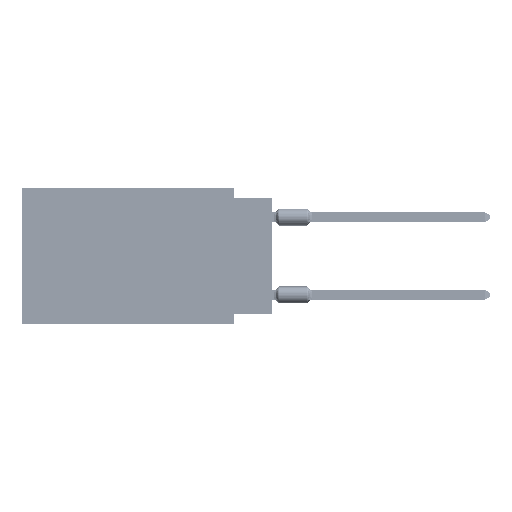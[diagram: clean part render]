
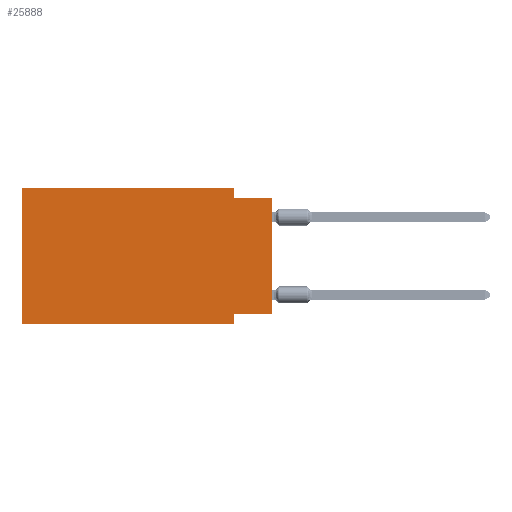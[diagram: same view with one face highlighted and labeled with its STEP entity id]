
A CAD part, left-side view. The second image highlights one B-rep face of the part: STEP entity #25888.
In plain terms, the highlighted planar face has unit normal (-1, 0, 0).
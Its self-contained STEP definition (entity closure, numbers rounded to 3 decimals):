
#6330 = VECTOR ( 'NONE', #55003, 1000. ) ;
#9241 = CARTESIAN_POINT ( 'NONE',  ( 0., 16.383, -8.89 ) ) ;
#10294 = EDGE_CURVE ( 'NONE', #30909, #75655, #40972, .T. ) ;
#11372 = ORIENTED_EDGE ( 'NONE', *, *, #43474, .F. ) ;
#11566 = LINE ( 'NONE', #36712, #68965 ) ;
#12037 = CARTESIAN_POINT ( 'NONE',  ( 0., 2.54, -8.89 ) ) ;
#12846 = LINE ( 'NONE', #12037, #32940 ) ;
#14534 = ORIENTED_EDGE ( 'NONE', *, *, #39581, .T. ) ;
#15841 = CARTESIAN_POINT ( 'NONE',  ( 0., 16.383, -8.89 ) ) ;
#17546 = VERTEX_POINT ( 'NONE', #73721 ) ;
#18106 = CARTESIAN_POINT ( 'NONE',  ( 0., 16.383, 0. ) ) ;
#19044 = VERTEX_POINT ( 'NONE', #76239 ) ;
#19432 = VERTEX_POINT ( 'NONE', #58290 ) ;
#19687 = LINE ( 'NONE', #53488, #44958 ) ;
#25888 = ADVANCED_FACE ( 'NONE', ( #49856 ), #80800, .F. ) ;
#26780 = VECTOR ( 'NONE', #71917, 1000. ) ;
#26903 = CARTESIAN_POINT ( 'NONE',  ( 0., 2.54, -8.89 ) ) ;
#28178 = CARTESIAN_POINT ( 'NONE',  ( 0., 16.383, 0. ) ) ;
#28678 = ORIENTED_EDGE ( 'NONE', *, *, #10294, .F. ) ;
#30092 = ORIENTED_EDGE ( 'NONE', *, *, #61820, .F. ) ;
#30909 = VERTEX_POINT ( 'NONE', #80794 ) ;
#31813 = DIRECTION ( 'NONE',  ( 0., 0., -1. ) ) ;
#32940 = VECTOR ( 'NONE', #31813, 1000. ) ;
#33059 = VECTOR ( 'NONE', #66560, 1000. ) ;
#33509 = CARTESIAN_POINT ( 'NONE',  ( 0., 16.383, 0. ) ) ;
#34720 = EDGE_CURVE ( 'NONE', #19432, #17546, #40091, .T. ) ;
#36712 = CARTESIAN_POINT ( 'NONE',  ( 0., 0., 0. ) ) ;
#38563 = DIRECTION ( 'NONE',  ( 0., -1., 0. ) ) ;
#38978 = VERTEX_POINT ( 'NONE', #26903 ) ;
#39581 = EDGE_CURVE ( 'NONE', #64849, #38978, #71942, .T. ) ;
#40091 = LINE ( 'NONE', #65261, #55985 ) ;
#40972 = LINE ( 'NONE', #66147, #33059 ) ;
#41267 = EDGE_LOOP ( 'NONE', ( #81431, #60183, #72199, #11372, #30092, #14534, #71300, #28678 ) ) ;
#43474 = EDGE_CURVE ( 'NONE', #45913, #19432, #19687, .T. ) ;
#43666 = DIRECTION ( 'NONE',  ( 0., 0., -1. ) ) ;
#44757 = CARTESIAN_POINT ( 'NONE',  ( 0., 0., -0.635 ) ) ;
#44958 = VECTOR ( 'NONE', #72061, 1000. ) ;
#45913 = VERTEX_POINT ( 'NONE', #33509 ) ;
#49856 = FACE_OUTER_BOUND ( 'NONE', #41267, .T. ) ;
#50536 = LINE ( 'NONE', #44757, #60083 ) ;
#53488 = CARTESIAN_POINT ( 'NONE',  ( 0., 16.383, 0. ) ) ;
#55003 = DIRECTION ( 'NONE',  ( 0., -1., 0. ) ) ;
#55685 = DIRECTION ( 'NONE',  ( 0., 0., 1. ) ) ;
#55985 = VECTOR ( 'NONE', #76825, 1000. ) ;
#58290 = CARTESIAN_POINT ( 'NONE',  ( 0., 2.54, 0. ) ) ;
#60073 = EDGE_CURVE ( 'NONE', #75655, #38978, #12846, .T. ) ;
#60083 = VECTOR ( 'NONE', #38563, 1000. ) ;
#60183 = ORIENTED_EDGE ( 'NONE', *, *, #68387, .F. ) ;
#61820 = EDGE_CURVE ( 'NONE', #64849, #45913, #64913, .T. ) ;
#62571 = EDGE_CURVE ( 'NONE', #30909, #19044, #11566, .T. ) ;
#64138 = AXIS2_PLACEMENT_3D ( 'NONE', #18106, #75041, #43666 ) ;
#64849 = VERTEX_POINT ( 'NONE', #15841 ) ;
#64913 = LINE ( 'NONE', #28178, #26780 ) ;
#65261 = CARTESIAN_POINT ( 'NONE',  ( 0., 2.54, 0. ) ) ;
#66147 = CARTESIAN_POINT ( 'NONE',  ( 0., 0., -8.255 ) ) ;
#66560 = DIRECTION ( 'NONE',  ( 0., 1., 0. ) ) ;
#68387 = EDGE_CURVE ( 'NONE', #17546, #19044, #50536, .T. ) ;
#68965 = VECTOR ( 'NONE', #55685, 1000. ) ;
#71300 = ORIENTED_EDGE ( 'NONE', *, *, #60073, .F. ) ;
#71917 = DIRECTION ( 'NONE',  ( 0., 0., 1. ) ) ;
#71942 = LINE ( 'NONE', #9241, #6330 ) ;
#72061 = DIRECTION ( 'NONE',  ( 0., -1., 0. ) ) ;
#72199 = ORIENTED_EDGE ( 'NONE', *, *, #34720, .F. ) ;
#73721 = CARTESIAN_POINT ( 'NONE',  ( 0., 2.54, -0.635 ) ) ;
#75041 = DIRECTION ( 'NONE',  ( 1., 0., 0. ) ) ;
#75655 = VERTEX_POINT ( 'NONE', #76981 ) ;
#76239 = CARTESIAN_POINT ( 'NONE',  ( 0., 0., -0.635 ) ) ;
#76825 = DIRECTION ( 'NONE',  ( 0., 0., -1. ) ) ;
#76981 = CARTESIAN_POINT ( 'NONE',  ( 0., 2.54, -8.255 ) ) ;
#80794 = CARTESIAN_POINT ( 'NONE',  ( 0., 0., -8.255 ) ) ;
#80800 = PLANE ( 'NONE',  #64138 ) ;
#81431 = ORIENTED_EDGE ( 'NONE', *, *, #62571, .T. ) ;
